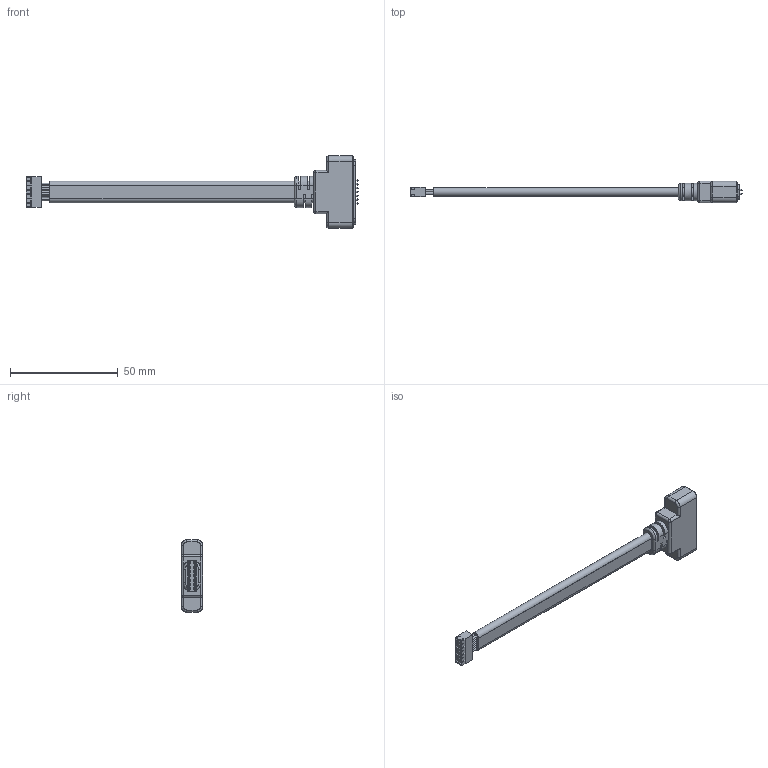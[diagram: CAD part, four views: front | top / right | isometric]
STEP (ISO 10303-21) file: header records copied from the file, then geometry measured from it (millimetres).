
FILE_DESCRIPTION (( 'STEP AP214' ), '1' );
FILE_NAME ('687B14224611100.STEP', '2023-04-13T15:48:41', ( '' ), ( '' ), 'SwSTEP 2.0', 'SolidWorks 2020', '' );
FILE_SCHEMA (( 'AUTOMOTIVE_DESIGN' ));
Length unit declared in the file: millimetre
Products named in the file (1): 687B14224611100
Bounding box: 154.25 x 9.9 x 33.6 mm (x, y, z)
Surface area: 7496.3 mm2 (no closed solid volume)
Topology: 0 solids, 2 shells, 726 faces, 1919 edges, 1132 vertices
Faces by surface type: plane 376, cylinder 220, torus 44, cone 36, sphere 36, bspline 14
Entity records: 31942 total; most frequent: CARTESIAN_POINT 8200, ORIENTED_EDGE 3550, DIRECTION 2759, EDGE_CURVE 1827, AXIS2_PLACEMENT_3D 1185, VERTEX_POINT 1090, B_SPLINE_CURVE_WITH_KNOTS 966, EDGE_LOOP 819
